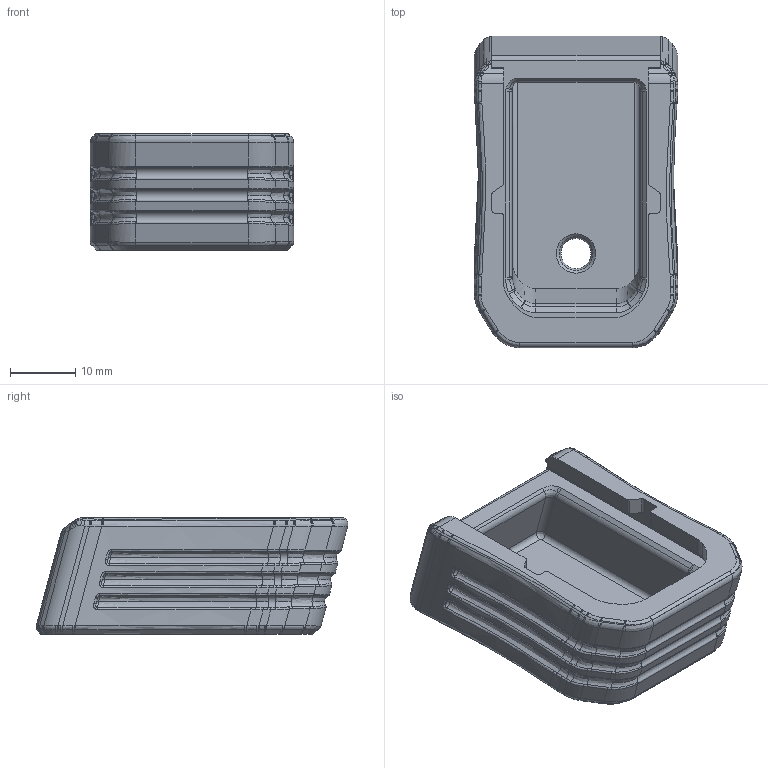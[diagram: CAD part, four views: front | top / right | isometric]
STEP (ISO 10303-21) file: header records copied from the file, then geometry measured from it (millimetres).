
FILE_DESCRIPTION(/* description */ (''),/* implementation_level */ '2;1');
FILE_NAME(/* name */ 'Final Concept.step',/* time_stamp */ '2021-06-16T23:27:09-04:00',/* author */ (''),/* organization */ (''),/* preprocessor_version */ 'ST-DEVELOPER v18.1',/* originating_system */ 'Autodesk Translation Framework v10.9.0.1377',/* authorisation */ '');
FILE_SCHEMA (('AUTOMOTIVE_DESIGN { 1 0 10303 214 3 1 1 }'));
Length unit declared in the file: millimetre
Products named in the file (1): +2 Dmg Extended Baseplate
Bounding box: 31.28 x 47.93 x 17.94 mm (x, y, z)
Volume: 11626.7 mm3; surface area: 6869.4 mm2
Topology: 1 solids, 1 shells, 778 faces, 1898 edges, 1124 vertices
Faces by surface type: bspline 509, cylinder 143, plane 90, torus 20, cone 16
Full cylindrical faces by diameter (mm): 4.64 x1
Entity records: 31655 total; most frequent: CARTESIAN_POINT 16294, ORIENTED_EDGE 3788, DIRECTION 2195, EDGE_CURVE 1894, VERTEX_POINT 1124, AXIS2_PLACEMENT_3D 868, B_SPLINE_CURVE_WITH_KNOTS 837, EDGE_LOOP 786
